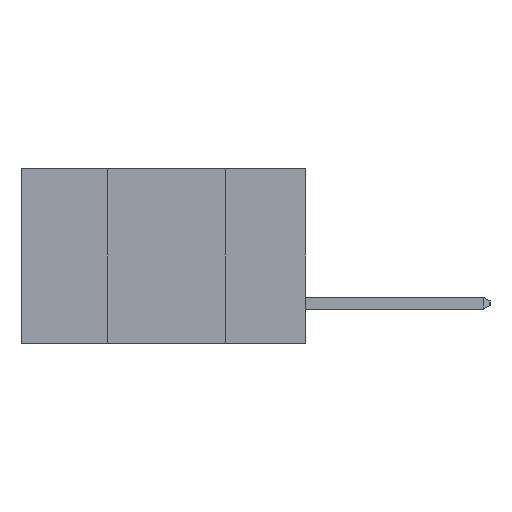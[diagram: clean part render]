
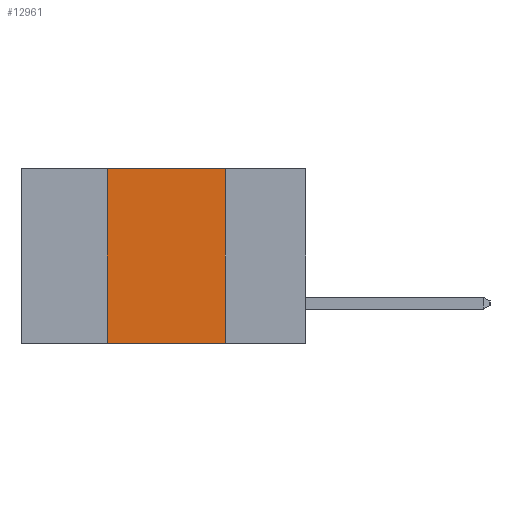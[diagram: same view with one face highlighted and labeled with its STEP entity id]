
A CAD part, left-side view. The second image highlights one B-rep face of the part: STEP entity #12961.
In plain terms, the highlighted planar face has unit normal (-1, 0, 0).
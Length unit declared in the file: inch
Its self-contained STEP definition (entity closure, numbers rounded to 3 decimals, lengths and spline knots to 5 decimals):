
#526 = EDGE_CURVE ( 'NONE', #2015, #2171, #7151, .T. ) ;
#677 = CARTESIAN_POINT ( 'NONE',  ( 0., 0.17, -0.37 ) ) ;
#1340 = DIRECTION ( 'NONE',  ( 1., 0., 0. ) ) ;
#1725 = VECTOR ( 'NONE', #2872, 39.37008 ) ;
#1773 = ORIENTED_EDGE ( 'NONE', *, *, #2430, .F. ) ;
#2015 = VERTEX_POINT ( 'NONE', #11977 ) ;
#2171 = VERTEX_POINT ( 'NONE', #12250 ) ;
#2430 = EDGE_CURVE ( 'NONE', #2171, #9980, #9373, .T. ) ;
#2872 = DIRECTION ( 'NONE',  ( 0., -1., 0. ) ) ;
#4147 = VECTOR ( 'NONE', #10221, 39.37008 ) ;
#4770 = CARTESIAN_POINT ( 'NONE',  ( 0., 0.6, 0. ) ) ;
#4771 = EDGE_LOOP ( 'NONE', ( #7326, #1773, #9053, #5498 ) ) ;
#5498 = ORIENTED_EDGE ( 'NONE', *, *, #6666, .T. ) ;
#5812 = VECTOR ( 'NONE', #12262, 39.37008 ) ;
#6666 = EDGE_CURVE ( 'NONE', #2015, #12050, #10340, .T. ) ;
#6889 = FACE_OUTER_BOUND ( 'NONE', #4771, .T. ) ;
#7151 = LINE ( 'NONE', #10674, #4147 ) ;
#7169 = CARTESIAN_POINT ( 'NONE',  ( 0., 0.17, 0. ) ) ;
#7326 = ORIENTED_EDGE ( 'NONE', *, *, #8743, .F. ) ;
#8147 = PLANE ( 'NONE',  #13012 ) ;
#8743 = EDGE_CURVE ( 'NONE', #9980, #12050, #11268, .T. ) ;
#9053 = ORIENTED_EDGE ( 'NONE', *, *, #526, .F. ) ;
#9282 = DIRECTION ( 'NONE',  ( 0., 0., -1. ) ) ;
#9373 = LINE ( 'NONE', #10697, #11833 ) ;
#9742 = CARTESIAN_POINT ( 'NONE',  ( 0., 0.6, -0.37 ) ) ;
#9980 = VERTEX_POINT ( 'NONE', #7169 ) ;
#10221 = DIRECTION ( 'NONE',  ( 0., 0., 1. ) ) ;
#10340 = LINE ( 'NONE', #9742, #1725 ) ;
#10674 = CARTESIAN_POINT ( 'NONE',  ( 0., 0.42, 0. ) ) ;
#10693 = DIRECTION ( 'NONE',  ( 0., -1., 0. ) ) ;
#10697 = CARTESIAN_POINT ( 'NONE',  ( 0., 0.6, 0. ) ) ;
#11268 = LINE ( 'NONE', #12277, #5812 ) ;
#11833 = VECTOR ( 'NONE', #10693, 39.37008 ) ;
#11977 = CARTESIAN_POINT ( 'NONE',  ( 0., 0.42, -0.37 ) ) ;
#12050 = VERTEX_POINT ( 'NONE', #677 ) ;
#12250 = CARTESIAN_POINT ( 'NONE',  ( 0., 0.42, 0. ) ) ;
#12262 = DIRECTION ( 'NONE',  ( 0., 0., -1. ) ) ;
#12277 = CARTESIAN_POINT ( 'NONE',  ( 0., 0.17, 0. ) ) ;
#12961 = ADVANCED_FACE ( 'NONE', ( #6889 ), #8147, .F. ) ;
#13012 = AXIS2_PLACEMENT_3D ( 'NONE', #4770, #1340, #9282 ) ;
